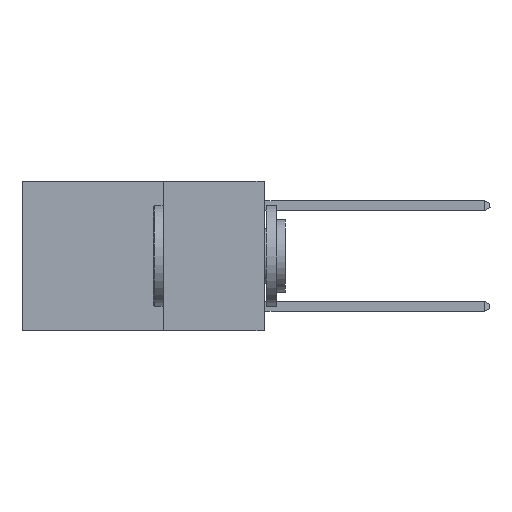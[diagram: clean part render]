
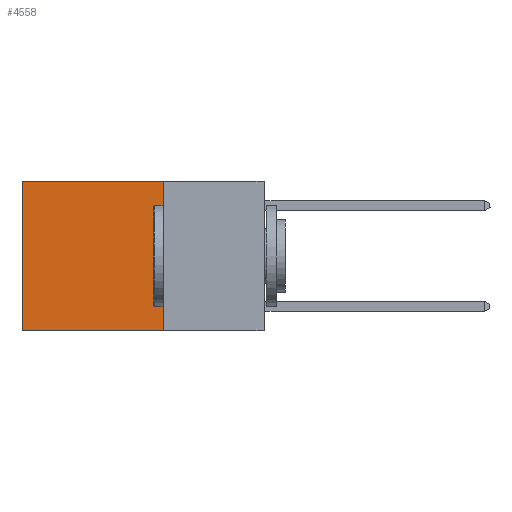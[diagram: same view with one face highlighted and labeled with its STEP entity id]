
A CAD part, left-side view. The second image highlights one B-rep face of the part: STEP entity #4558.
In plain terms, the highlighted planar face has unit normal (-1, 0, 0).
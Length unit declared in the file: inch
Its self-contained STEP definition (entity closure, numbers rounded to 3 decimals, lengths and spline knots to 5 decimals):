
#467 = DIRECTION ( 'NONE',  ( 1., 0., 0. ) ) ;
#605 = CARTESIAN_POINT ( 'NONE',  ( 0.2625, 0.25, 0. ) ) ;
#993 = LINE ( 'NONE', #12944, #5917 ) ;
#2247 = VECTOR ( 'NONE', #13766, 39.37008 ) ;
#2735 = EDGE_CURVE ( 'NONE', #12769, #6806, #8396, .T. ) ;
#3165 = CARTESIAN_POINT ( 'NONE',  ( 0.2625, 0.6, 0. ) ) ;
#3823 = ORIENTED_EDGE ( 'NONE', *, *, #14038, .F. ) ;
#3828 = CARTESIAN_POINT ( 'NONE',  ( 0.2625, 0.25, 0. ) ) ;
#4558 = ADVANCED_FACE ( 'NONE', ( #11906 ), #9323, .F. ) ;
#4757 = ORIENTED_EDGE ( 'NONE', *, *, #11275, .T. ) ;
#5817 = ORIENTED_EDGE ( 'NONE', *, *, #7739, .F. ) ;
#5917 = VECTOR ( 'NONE', #6425, 39.37008 ) ;
#6425 = DIRECTION ( 'NONE',  ( 0., 1., 0. ) ) ;
#6806 = VERTEX_POINT ( 'NONE', #7716 ) ;
#7716 = CARTESIAN_POINT ( 'NONE',  ( 0.2625, 0.6, -0.37 ) ) ;
#7739 = EDGE_CURVE ( 'NONE', #8645, #6806, #13856, .T. ) ;
#7908 = VECTOR ( 'NONE', #10886, 39.37008 ) ;
#8083 = CARTESIAN_POINT ( 'NONE',  ( 0.2625, 0.25, 0. ) ) ;
#8396 = LINE ( 'NONE', #9776, #7908 ) ;
#8645 = VERTEX_POINT ( 'NONE', #10918 ) ;
#8783 = VECTOR ( 'NONE', #11308, 39.37008 ) ;
#9323 = PLANE ( 'NONE',  #13934 ) ;
#9776 = CARTESIAN_POINT ( 'NONE',  ( 0.2625, 0.6, 0. ) ) ;
#9862 = CARTESIAN_POINT ( 'NONE',  ( 0.2625, 0.25, -0.37 ) ) ;
#9974 = ORIENTED_EDGE ( 'NONE', *, *, #2735, .T. ) ;
#10164 = VERTEX_POINT ( 'NONE', #8083 ) ;
#10886 = DIRECTION ( 'NONE',  ( 0., 0., -1. ) ) ;
#10918 = CARTESIAN_POINT ( 'NONE',  ( 0.2625, 0.25, -0.37 ) ) ;
#10957 = LINE ( 'NONE', #3828, #2247 ) ;
#11247 = EDGE_LOOP ( 'NONE', ( #9974, #5817, #3823, #4757 ) ) ;
#11275 = EDGE_CURVE ( 'NONE', #10164, #12769, #993, .T. ) ;
#11308 = DIRECTION ( 'NONE',  ( 0., 1., 0. ) ) ;
#11906 = FACE_OUTER_BOUND ( 'NONE', #11247, .T. ) ;
#12769 = VERTEX_POINT ( 'NONE', #3165 ) ;
#12944 = CARTESIAN_POINT ( 'NONE',  ( 0.2625, 0.25, 0. ) ) ;
#13693 = DIRECTION ( 'NONE',  ( 0., 0., -1. ) ) ;
#13766 = DIRECTION ( 'NONE',  ( 0., 0., -1. ) ) ;
#13856 = LINE ( 'NONE', #9862, #8783 ) ;
#13934 = AXIS2_PLACEMENT_3D ( 'NONE', #605, #467, #13693 ) ;
#14038 = EDGE_CURVE ( 'NONE', #10164, #8645, #10957, .T. ) ;
